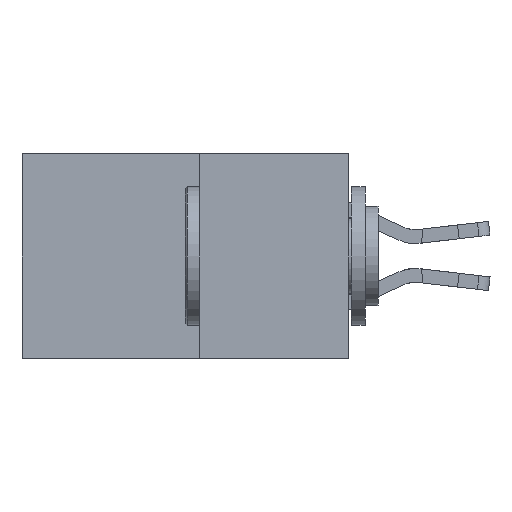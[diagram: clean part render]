
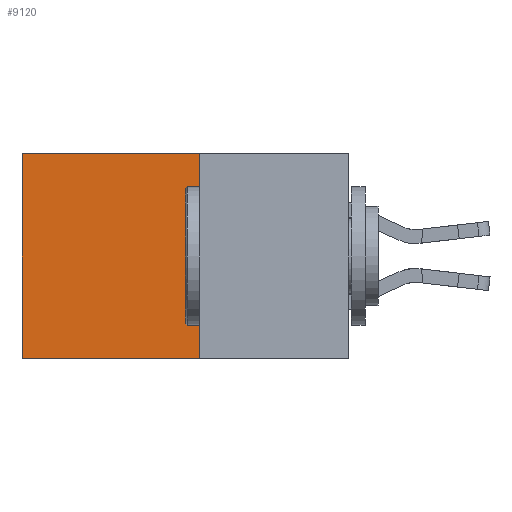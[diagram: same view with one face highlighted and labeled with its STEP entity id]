
A CAD part, left-side view. The second image highlights one B-rep face of the part: STEP entity #9120.
In plain terms, the highlighted planar face has unit normal (-1, 0, 0).
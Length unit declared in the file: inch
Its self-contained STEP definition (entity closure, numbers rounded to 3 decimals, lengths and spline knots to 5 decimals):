
#195 = ORIENTED_EDGE ( 'NONE', *, *, #21456, .F. ) ;
#778 = VECTOR ( 'NONE', #1997, 39.37008 ) ;
#1927 = CARTESIAN_POINT ( 'NONE',  ( 0.277, 0.27, -0.37 ) ) ;
#1997 = DIRECTION ( 'NONE',  ( 0., 1., 0. ) ) ;
#5310 = CARTESIAN_POINT ( 'NONE',  ( 0.277, 0.27, -0.37 ) ) ;
#5893 = ORIENTED_EDGE ( 'NONE', *, *, #19338, .F. ) ;
#6247 = DIRECTION ( 'NONE',  ( 0., 0., -1. ) ) ;
#7140 = EDGE_CURVE ( 'NONE', #19697, #8858, #16672, .T. ) ;
#8844 = VERTEX_POINT ( 'NONE', #5310 ) ;
#8858 = VERTEX_POINT ( 'NONE', #24747 ) ;
#9063 = LINE ( 'NONE', #11811, #19851 ) ;
#9120 = ADVANCED_FACE ( 'NONE', ( #9315 ), #17043, .F. ) ;
#9315 = FACE_OUTER_BOUND ( 'NONE', #14354, .T. ) ;
#10489 = CARTESIAN_POINT ( 'NONE',  ( 0.277, 0.27, -0.37 ) ) ;
#11811 = CARTESIAN_POINT ( 'NONE',  ( 0.277, 0.27, -0.37 ) ) ;
#11946 = VERTEX_POINT ( 'NONE', #18659 ) ;
#12749 = CARTESIAN_POINT ( 'NONE',  ( 0.277, 0.27, 0. ) ) ;
#14000 = DIRECTION ( 'NONE',  ( 0., 1., 0. ) ) ;
#14048 = LINE ( 'NONE', #16813, #25468 ) ;
#14354 = EDGE_LOOP ( 'NONE', ( #16897, #195, #5893, #24760 ) ) ;
#16672 = LINE ( 'NONE', #12749, #778 ) ;
#16813 = CARTESIAN_POINT ( 'NONE',  ( 0.277, 0.59, -0.37 ) ) ;
#16897 = ORIENTED_EDGE ( 'NONE', *, *, #23768, .T. ) ;
#16938 = AXIS2_PLACEMENT_3D ( 'NONE', #1927, #19173, #6247 ) ;
#17043 = PLANE ( 'NONE',  #16938 ) ;
#17939 = CARTESIAN_POINT ( 'NONE',  ( 0.277, 0.27, 0. ) ) ;
#18659 = CARTESIAN_POINT ( 'NONE',  ( 0.277, 0.59, -0.37 ) ) ;
#18953 = DIRECTION ( 'NONE',  ( 0., 0., -1. ) ) ;
#19173 = DIRECTION ( 'NONE',  ( 1., 0., 0. ) ) ;
#19338 = EDGE_CURVE ( 'NONE', #19697, #8844, #27724, .T. ) ;
#19697 = VERTEX_POINT ( 'NONE', #17939 ) ;
#19851 = VECTOR ( 'NONE', #14000, 39.37008 ) ;
#21322 = VECTOR ( 'NONE', #25560, 39.37008 ) ;
#21456 = EDGE_CURVE ( 'NONE', #8844, #11946, #9063, .T. ) ;
#23768 = EDGE_CURVE ( 'NONE', #8858, #11946, #14048, .T. ) ;
#24747 = CARTESIAN_POINT ( 'NONE',  ( 0.277, 0.59, 0. ) ) ;
#24760 = ORIENTED_EDGE ( 'NONE', *, *, #7140, .T. ) ;
#25468 = VECTOR ( 'NONE', #18953, 39.37008 ) ;
#25560 = DIRECTION ( 'NONE',  ( 0., 0., -1. ) ) ;
#27724 = LINE ( 'NONE', #10489, #21322 ) ;
